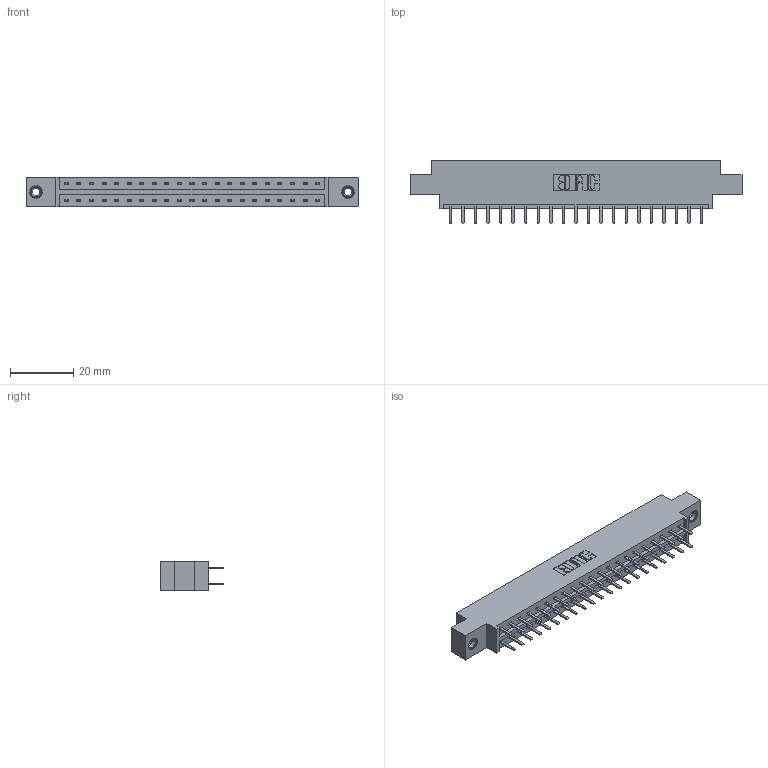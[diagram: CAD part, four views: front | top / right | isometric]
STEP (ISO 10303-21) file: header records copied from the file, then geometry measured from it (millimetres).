
FILE_DESCRIPTION (( 'STEP AP203' ), '1' );
FILE_NAME ('333-042-520-808.STEP', '2018-08-03T17:26:25', ( '' ), ( '' ), 'SwSTEP 2.0', 'SolidWorks 2016', '' );
FILE_SCHEMA (( 'CONFIG_CONTROL_DESIGN' ));
Length unit declared in the file: inch
Products named in the file (4): 333 Part_Offset - .156 Dia - TI; 345-292-001_345-293-120; 345-250-001_345-250-003-102; 333-042-520-808
Assembly tree (45 placements, depth 2):
  333-042-520-808
    333 Part_Offset - .156 Dia - TI
    345-292-001_345-293-120  x42
    345-250-001_345-250-003-102  x2
Bounding box: 104.75 x 20.02 x 9.4 mm (x, y, z)
Volume: 10245.2 mm3; surface area: 12080.4 mm2
Topology: 45 solids, 45 shells, 2530 faces, 7305 edges, 4750 vertices
Faces by surface type: plane 1702, cylinder 812, cone 12, torus 4
Entity records: 17658 total; most frequent: CARTESIAN_POINT 2949, ORIENTED_EDGE 2866, DIRECTION 2575, EDGE_CURVE 1433, LINE 1281, VECTOR 1281, VERTEX_POINT 948, AXIS2_PLACEMENT_3D 647
